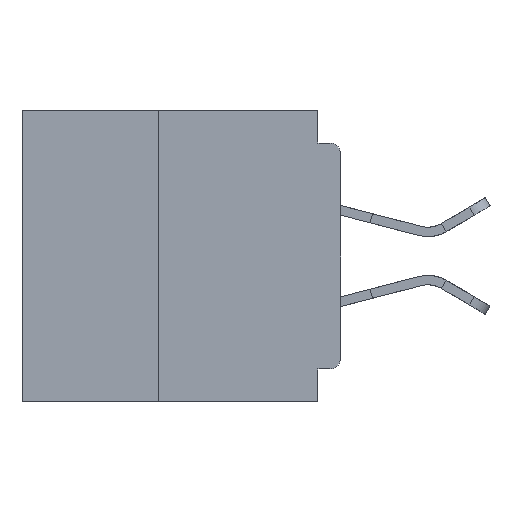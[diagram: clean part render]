
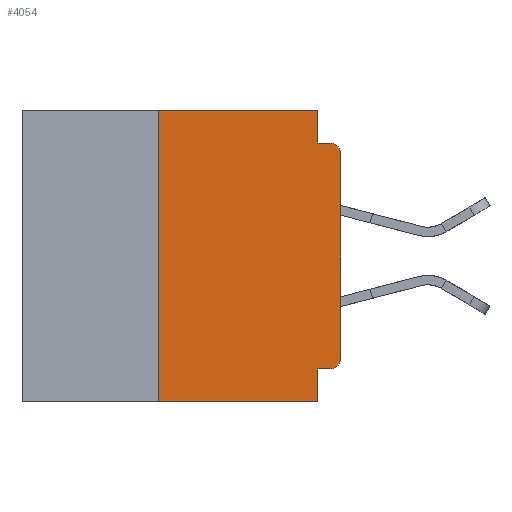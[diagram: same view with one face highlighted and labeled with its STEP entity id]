
A CAD part, left-side view. The second image highlights one B-rep face of the part: STEP entity #4054.
In plain terms, the highlighted planar face has unit normal (-1, 0, 0).
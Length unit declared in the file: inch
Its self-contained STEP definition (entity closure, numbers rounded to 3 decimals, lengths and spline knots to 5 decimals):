
#41 = EDGE_CURVE ( 'NONE', #23488, #16118, #9899, .T. ) ;
#814 = VECTOR ( 'NONE', #27406, 39.37008 ) ;
#864 = ORIENTED_EDGE ( 'NONE', *, *, #14658, .F. ) ;
#953 = CARTESIAN_POINT ( 'NONE',  ( 0., 0.031, 0. ) ) ;
#1047 = ORIENTED_EDGE ( 'NONE', *, *, #17121, .T. ) ;
#1538 = VERTEX_POINT ( 'NONE', #12367 ) ;
#1901 = LINE ( 'NONE', #13444, #814 ) ;
#3113 = CARTESIAN_POINT ( 'NONE',  ( 0., 0., -0.355 ) ) ;
#3614 = VECTOR ( 'NONE', #11918, 39.37008 ) ;
#3677 = CARTESIAN_POINT ( 'NONE',  ( 0., 0.015, -0.355 ) ) ;
#3897 = EDGE_CURVE ( 'NONE', #23488, #9254, #33972, .T. ) ;
#3926 = LINE ( 'NONE', #953, #23465 ) ;
#4054 = ADVANCED_FACE ( 'NONE', ( #19282 ), #31638, .F. ) ;
#4440 = VERTEX_POINT ( 'NONE', #26752 ) ;
#4778 = CARTESIAN_POINT ( 'NONE',  ( 0., 0., 0. ) ) ;
#6348 = VERTEX_POINT ( 'NONE', #32485 ) ;
#8196 = LINE ( 'NONE', #4778, #26604 ) ;
#8312 = DIRECTION ( 'NONE',  ( 0., 0., 1. ) ) ;
#9254 = VERTEX_POINT ( 'NONE', #30553 ) ;
#9530 = DIRECTION ( 'NONE',  ( 0., -1., 0. ) ) ;
#9899 = CIRCLE ( 'NONE', #39698, 0.015 ) ;
#10845 = EDGE_CURVE ( 'NONE', #6348, #24197, #3926, .T. ) ;
#10894 = CARTESIAN_POINT ( 'NONE',  ( 0., 0.437, 0. ) ) ;
#11011 = CARTESIAN_POINT ( 'NONE',  ( 0., 0.031, -0.4 ) ) ;
#11349 = DIRECTION ( 'NONE',  ( 0., 0., -1. ) ) ;
#11918 = DIRECTION ( 'NONE',  ( 0., 0., -1. ) ) ;
#12367 = CARTESIAN_POINT ( 'NONE',  ( 0., 0.015, -0.045 ) ) ;
#13124 = VERTEX_POINT ( 'NONE', #11011 ) ;
#13279 = VECTOR ( 'NONE', #25291, 39.37008 ) ;
#13444 = CARTESIAN_POINT ( 'NONE',  ( 0., 0.25, -0.4 ) ) ;
#13453 = DIRECTION ( 'NONE',  ( -1., 0., 0. ) ) ;
#14116 = VERTEX_POINT ( 'NONE', #24558 ) ;
#14338 = DIRECTION ( 'NONE',  ( 0., 0., -1. ) ) ;
#14658 = EDGE_CURVE ( 'NONE', #4440, #14116, #1901, .T. ) ;
#14716 = CARTESIAN_POINT ( 'NONE',  ( 0., 0.031, -0.045 ) ) ;
#14861 = ORIENTED_EDGE ( 'NONE', *, *, #10845, .F. ) ;
#14972 = CARTESIAN_POINT ( 'NONE',  ( 0., 0.437, -0.4 ) ) ;
#15014 = CARTESIAN_POINT ( 'NONE',  ( 0., 0., -0.34 ) ) ;
#16118 = VERTEX_POINT ( 'NONE', #15014 ) ;
#16712 = ORIENTED_EDGE ( 'NONE', *, *, #40566, .F. ) ;
#16854 = CARTESIAN_POINT ( 'NONE',  ( 0., 0., -0.045 ) ) ;
#17121 = EDGE_CURVE ( 'NONE', #39678, #1538, #30059, .T. ) ;
#19282 = FACE_OUTER_BOUND ( 'NONE', #30247, .T. ) ;
#20078 = ORIENTED_EDGE ( 'NONE', *, *, #43713, .T. ) ;
#20956 = LINE ( 'NONE', #36174, #3614 ) ;
#23024 = EDGE_CURVE ( 'NONE', #4440, #13124, #42018, .T. ) ;
#23465 = VECTOR ( 'NONE', #11349, 39.37008 ) ;
#23488 = VERTEX_POINT ( 'NONE', #3677 ) ;
#23827 = CARTESIAN_POINT ( 'NONE',  ( 0., 0.015, -0.34 ) ) ;
#23893 = ORIENTED_EDGE ( 'NONE', *, *, #41, .T. ) ;
#23932 = EDGE_CURVE ( 'NONE', #24197, #1538, #35231, .T. ) ;
#24197 = VERTEX_POINT ( 'NONE', #14716 ) ;
#24483 = DIRECTION ( 'NONE',  ( -1., 0., 0. ) ) ;
#24489 = DIRECTION ( 'NONE',  ( 0., 0., -1. ) ) ;
#24558 = CARTESIAN_POINT ( 'NONE',  ( 0., 0.25, 0. ) ) ;
#25291 = DIRECTION ( 'NONE',  ( 0., -1., 0. ) ) ;
#26604 = VECTOR ( 'NONE', #8312, 39.37008 ) ;
#26752 = CARTESIAN_POINT ( 'NONE',  ( 0., 0.25, -0.4 ) ) ;
#27406 = DIRECTION ( 'NONE',  ( 0., 0., 1. ) ) ;
#27973 = AXIS2_PLACEMENT_3D ( 'NONE', #10894, #35133, #14338 ) ;
#30059 = CIRCLE ( 'NONE', #34254, 0.015 ) ;
#30103 = CARTESIAN_POINT ( 'NONE',  ( 0., 0.437, 0. ) ) ;
#30247 = EDGE_LOOP ( 'NONE', ( #20078, #1047, #42151, #14861, #34759, #864, #35357, #16712, #42536, #23893 ) ) ;
#30553 = CARTESIAN_POINT ( 'NONE',  ( 0., 0.031, -0.355 ) ) ;
#30843 = EDGE_CURVE ( 'NONE', #14116, #6348, #40918, .T. ) ;
#30886 = DIRECTION ( 'NONE',  ( 0., 1., 0. ) ) ;
#31498 = CARTESIAN_POINT ( 'NONE',  ( 0., 0., -0.06 ) ) ;
#31638 = PLANE ( 'NONE',  #27973 ) ;
#32485 = CARTESIAN_POINT ( 'NONE',  ( 0., 0.031, 0. ) ) ;
#33972 = LINE ( 'NONE', #3113, #44236 ) ;
#34250 = CARTESIAN_POINT ( 'NONE',  ( 0., 0.015, -0.06 ) ) ;
#34254 = AXIS2_PLACEMENT_3D ( 'NONE', #34250, #13453, #37734 ) ;
#34759 = ORIENTED_EDGE ( 'NONE', *, *, #30843, .F. ) ;
#35133 = DIRECTION ( 'NONE',  ( 1., 0., 0. ) ) ;
#35231 = LINE ( 'NONE', #16854, #43317 ) ;
#35357 = ORIENTED_EDGE ( 'NONE', *, *, #23024, .T. ) ;
#36174 = CARTESIAN_POINT ( 'NONE',  ( 0., 0.031, -0.4 ) ) ;
#37734 = DIRECTION ( 'NONE',  ( 0., 0., -1. ) ) ;
#39678 = VERTEX_POINT ( 'NONE', #31498 ) ;
#39698 = AXIS2_PLACEMENT_3D ( 'NONE', #23827, #24483, #24489 ) ;
#40566 = EDGE_CURVE ( 'NONE', #9254, #13124, #20956, .T. ) ;
#40918 = LINE ( 'NONE', #30103, #43911 ) ;
#42018 = LINE ( 'NONE', #14972, #13279 ) ;
#42151 = ORIENTED_EDGE ( 'NONE', *, *, #23932, .F. ) ;
#42536 = ORIENTED_EDGE ( 'NONE', *, *, #3897, .F. ) ;
#43317 = VECTOR ( 'NONE', #44566, 39.37008 ) ;
#43713 = EDGE_CURVE ( 'NONE', #16118, #39678, #8196, .T. ) ;
#43911 = VECTOR ( 'NONE', #9530, 39.37008 ) ;
#44236 = VECTOR ( 'NONE', #30886, 39.37008 ) ;
#44566 = DIRECTION ( 'NONE',  ( 0., -1., 0. ) ) ;
